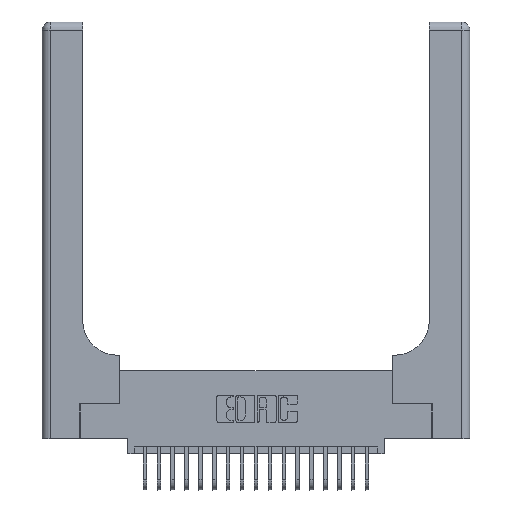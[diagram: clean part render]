
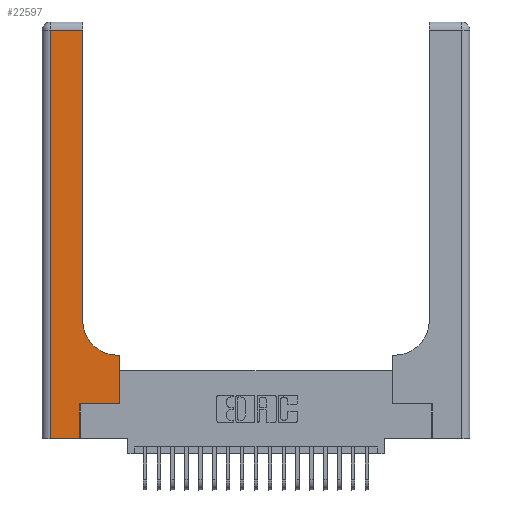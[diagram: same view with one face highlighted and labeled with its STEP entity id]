
A CAD part, top view. The second image highlights one B-rep face of the part: STEP entity #22597.
In plain terms, the highlighted planar face has unit normal (0, 0, 1).
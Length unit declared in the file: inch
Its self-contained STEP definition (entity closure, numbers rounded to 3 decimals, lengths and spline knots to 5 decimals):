
#53 = LINE ( 'NONE', #19135, #22162 ) ;
#419 = VERTEX_POINT ( 'NONE', #18989 ) ;
#880 = VERTEX_POINT ( 'NONE', #8988 ) ;
#1829 = CARTESIAN_POINT ( 'NONE',  ( 0.2915, 0.6, 0.37 ) ) ;
#2130 = CARTESIAN_POINT ( 'NONE',  ( 0.06, 0., 0.37 ) ) ;
#2784 = VECTOR ( 'NONE', #7277, 39.37008 ) ;
#2795 = CARTESIAN_POINT ( 'NONE',  ( 0., 3., 0.37 ) ) ;
#2979 = EDGE_CURVE ( 'NONE', #880, #7531, #21757, .T. ) ;
#3109 = CARTESIAN_POINT ( 'NONE',  ( 0.5415, 0.6, 0.37 ) ) ;
#3177 = CARTESIAN_POINT ( 'NONE',  ( 0., 0., 0.37 ) ) ;
#3287 = FACE_OUTER_BOUND ( 'NONE', #7761, .T. ) ;
#3339 = CARTESIAN_POINT ( 'NONE',  ( 0.06, 3., 0.37 ) ) ;
#3661 = VECTOR ( 'NONE', #7519, 39.37008 ) ;
#4050 = VERTEX_POINT ( 'NONE', #12370 ) ;
#4670 = DIRECTION ( 'NONE',  ( -1., 0., 0. ) ) ;
#5078 = ORIENTED_EDGE ( 'NONE', *, *, #14551, .T. ) ;
#5294 = ORIENTED_EDGE ( 'NONE', *, *, #19754, .T. ) ;
#5508 = CARTESIAN_POINT ( 'NONE',  ( 0.269, 0.25, 0.37 ) ) ;
#5591 = VECTOR ( 'NONE', #10547, 39.37008 ) ;
#6168 = LINE ( 'NONE', #16016, #5591 ) ;
#6568 = EDGE_CURVE ( 'NONE', #19940, #880, #53, .T. ) ;
#6882 = EDGE_CURVE ( 'NONE', #4050, #23265, #13217, .T. ) ;
#6921 = EDGE_CURVE ( 'NONE', #11522, #419, #8301, .T. ) ;
#7277 = DIRECTION ( 'NONE',  ( 0., 1., 0. ) ) ;
#7342 = DIRECTION ( 'NONE',  ( -1., 0., 0. ) ) ;
#7519 = DIRECTION ( 'NONE',  ( 0., 1., 0. ) ) ;
#7531 = VERTEX_POINT ( 'NONE', #2130 ) ;
#7761 = EDGE_LOOP ( 'NONE', ( #11941, #9758, #12757, #20008, #18615, #5078, #16150, #5294, #23325 ) ) ;
#8301 = CIRCLE ( 'NONE', #22668, 0.25 ) ;
#8771 = DIRECTION ( 'NONE',  ( 1., 0., 0. ) ) ;
#8988 = CARTESIAN_POINT ( 'NONE',  ( 0.06, 2.94, 0.37 ) ) ;
#9220 = DIRECTION ( 'NONE',  ( 0., 0., -1. ) ) ;
#9676 = CARTESIAN_POINT ( 'NONE',  ( 0.2915, 2.94, 0.37 ) ) ;
#9758 = ORIENTED_EDGE ( 'NONE', *, *, #6568, .T. ) ;
#10547 = DIRECTION ( 'NONE',  ( 0., 1., 0. ) ) ;
#11522 = VERTEX_POINT ( 'NONE', #3109 ) ;
#11941 = ORIENTED_EDGE ( 'NONE', *, *, #23380, .T. ) ;
#12041 = PLANE ( 'NONE',  #13004 ) ;
#12370 = CARTESIAN_POINT ( 'NONE',  ( 0.5585, 0.25, 0.37 ) ) ;
#12657 = DIRECTION ( 'NONE',  ( 0., -1., 0. ) ) ;
#12757 = ORIENTED_EDGE ( 'NONE', *, *, #2979, .T. ) ;
#13004 = AXIS2_PLACEMENT_3D ( 'NONE', #2795, #15721, #4670 ) ;
#13217 = LINE ( 'NONE', #18270, #2784 ) ;
#13949 = CARTESIAN_POINT ( 'NONE',  ( 0.5585, 0.6, 0.37 ) ) ;
#14551 = EDGE_CURVE ( 'NONE', #20464, #4050, #16544, .T. ) ;
#15721 = DIRECTION ( 'NONE',  ( 0., 0., -1. ) ) ;
#16016 = CARTESIAN_POINT ( 'NONE',  ( 0.2915, 3., 0.37 ) ) ;
#16150 = ORIENTED_EDGE ( 'NONE', *, *, #6882, .T. ) ;
#16544 = LINE ( 'NONE', #5508, #21838 ) ;
#16681 = VERTEX_POINT ( 'NONE', #17211 ) ;
#17018 = VECTOR ( 'NONE', #12657, 39.37008 ) ;
#17211 = CARTESIAN_POINT ( 'NONE',  ( 0.269, 0., 0.37 ) ) ;
#18270 = CARTESIAN_POINT ( 'NONE',  ( 0.5585, 0.25, 0.37 ) ) ;
#18288 = VECTOR ( 'NONE', #7342, 39.37008 ) ;
#18364 = LINE ( 'NONE', #20299, #3661 ) ;
#18370 = DIRECTION ( 'NONE',  ( 1., 0., 0. ) ) ;
#18541 = CARTESIAN_POINT ( 'NONE',  ( 0.269, 0.25, 0.37 ) ) ;
#18615 = ORIENTED_EDGE ( 'NONE', *, *, #21035, .T. ) ;
#18838 = LINE ( 'NONE', #1829, #18288 ) ;
#18989 = CARTESIAN_POINT ( 'NONE',  ( 0.2915, 0.85, 0.37 ) ) ;
#19135 = CARTESIAN_POINT ( 'NONE',  ( 0., 2.94, 0.37 ) ) ;
#19424 = LINE ( 'NONE', #3177, #22420 ) ;
#19754 = EDGE_CURVE ( 'NONE', #23265, #11522, #18838, .T. ) ;
#19940 = VERTEX_POINT ( 'NONE', #9676 ) ;
#20008 = ORIENTED_EDGE ( 'NONE', *, *, #21921, .T. ) ;
#20145 = CARTESIAN_POINT ( 'NONE',  ( 0.5415, 0.85, 0.37 ) ) ;
#20299 = CARTESIAN_POINT ( 'NONE',  ( 0.269, 0., 0.37 ) ) ;
#20464 = VERTEX_POINT ( 'NONE', #18541 ) ;
#20921 = DIRECTION ( 'NONE',  ( -1., 0., 0. ) ) ;
#21035 = EDGE_CURVE ( 'NONE', #16681, #20464, #18364, .T. ) ;
#21757 = LINE ( 'NONE', #3339, #17018 ) ;
#21838 = VECTOR ( 'NONE', #18370, 39.37008 ) ;
#21886 = DIRECTION ( 'NONE',  ( 1., 0., 0. ) ) ;
#21921 = EDGE_CURVE ( 'NONE', #7531, #16681, #19424, .T. ) ;
#22162 = VECTOR ( 'NONE', #20921, 39.37008 ) ;
#22420 = VECTOR ( 'NONE', #8771, 39.37008 ) ;
#22597 = ADVANCED_FACE ( 'NONE', ( #3287 ), #12041, .F. ) ;
#22668 = AXIS2_PLACEMENT_3D ( 'NONE', #20145, #9220, #21886 ) ;
#23265 = VERTEX_POINT ( 'NONE', #13949 ) ;
#23325 = ORIENTED_EDGE ( 'NONE', *, *, #6921, .T. ) ;
#23380 = EDGE_CURVE ( 'NONE', #419, #19940, #6168, .T. ) ;
